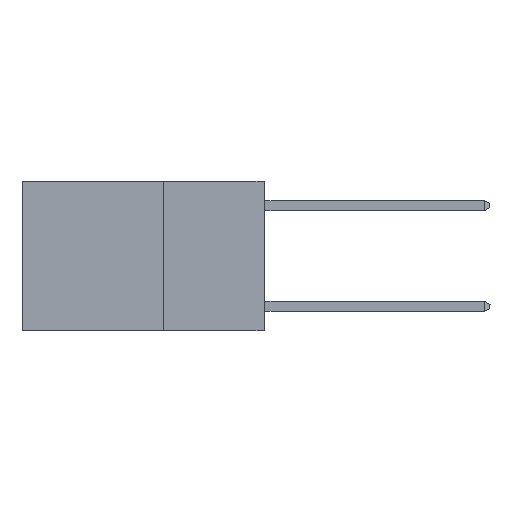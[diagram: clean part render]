
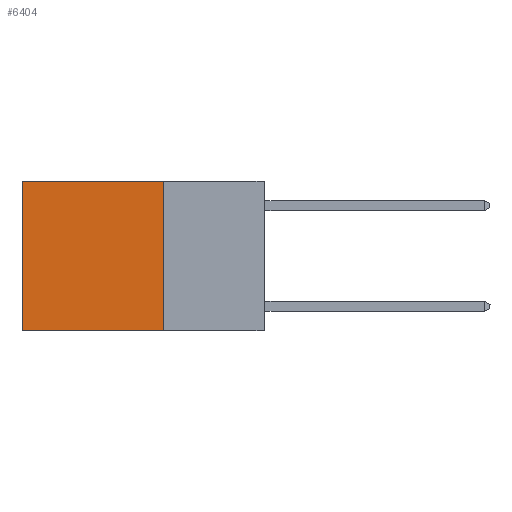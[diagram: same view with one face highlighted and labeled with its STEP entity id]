
A CAD part, left-side view. The second image highlights one B-rep face of the part: STEP entity #6404.
In plain terms, the highlighted planar face has unit normal (-1, 0, 0).
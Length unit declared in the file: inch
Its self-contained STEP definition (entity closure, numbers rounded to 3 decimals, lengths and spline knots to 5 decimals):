
#98 = EDGE_CURVE ( 'NONE', #1555, #681, #8851, .T. ) ;
#681 = VERTEX_POINT ( 'NONE', #6978 ) ;
#824 = EDGE_LOOP ( 'NONE', ( #1961, #2240, #9434, #9918 ) ) ;
#958 = VERTEX_POINT ( 'NONE', #6977 ) ;
#1031 = DIRECTION ( 'NONE',  ( 0., 0., -1. ) ) ;
#1322 = EDGE_CURVE ( 'NONE', #7547, #1555, #7709, .T. ) ;
#1414 = CARTESIAN_POINT ( 'NONE',  ( 0.2625, 0.6, 0. ) ) ;
#1555 = VERTEX_POINT ( 'NONE', #6899 ) ;
#1961 = ORIENTED_EDGE ( 'NONE', *, *, #9057, .T. ) ;
#2240 = ORIENTED_EDGE ( 'NONE', *, *, #98, .F. ) ;
#2526 = CARTESIAN_POINT ( 'NONE',  ( 0.2625, 0.25, -0.37 ) ) ;
#3001 = CARTESIAN_POINT ( 'NONE',  ( 0.2625, 0.25, 0. ) ) ;
#3816 = VECTOR ( 'NONE', #6089, 39.37008 ) ;
#4702 = CARTESIAN_POINT ( 'NONE',  ( 0.2625, 0.25, 0. ) ) ;
#4886 = VECTOR ( 'NONE', #12712, 39.37008 ) ;
#5017 = PLANE ( 'NONE',  #7343 ) ;
#5266 = VECTOR ( 'NONE', #12694, 39.37008 ) ;
#6089 = DIRECTION ( 'NONE',  ( 0., 1., 0. ) ) ;
#6404 = ADVANCED_FACE ( 'NONE', ( #6633 ), #5017, .F. ) ;
#6525 = LINE ( 'NONE', #12337, #3816 ) ;
#6633 = FACE_OUTER_BOUND ( 'NONE', #824, .T. ) ;
#6899 = CARTESIAN_POINT ( 'NONE',  ( 0.2625, 0.25, -0.37 ) ) ;
#6977 = CARTESIAN_POINT ( 'NONE',  ( 0.2625, 0.6, 0. ) ) ;
#6978 = CARTESIAN_POINT ( 'NONE',  ( 0.2625, 0.6, -0.37 ) ) ;
#7101 = DIRECTION ( 'NONE',  ( 1., 0., 0. ) ) ;
#7343 = AXIS2_PLACEMENT_3D ( 'NONE', #3001, #7101, #1031 ) ;
#7547 = VERTEX_POINT ( 'NONE', #4702 ) ;
#7688 = VECTOR ( 'NONE', #11388, 39.37008 ) ;
#7709 = LINE ( 'NONE', #11270, #7688 ) ;
#8263 = EDGE_CURVE ( 'NONE', #7547, #958, #6525, .T. ) ;
#8851 = LINE ( 'NONE', #2526, #4886 ) ;
#9057 = EDGE_CURVE ( 'NONE', #958, #681, #10827, .T. ) ;
#9434 = ORIENTED_EDGE ( 'NONE', *, *, #1322, .F. ) ;
#9918 = ORIENTED_EDGE ( 'NONE', *, *, #8263, .T. ) ;
#10827 = LINE ( 'NONE', #1414, #5266 ) ;
#11270 = CARTESIAN_POINT ( 'NONE',  ( 0.2625, 0.25, 0. ) ) ;
#11388 = DIRECTION ( 'NONE',  ( 0., 0., -1. ) ) ;
#12337 = CARTESIAN_POINT ( 'NONE',  ( 0.2625, 0.25, 0. ) ) ;
#12694 = DIRECTION ( 'NONE',  ( 0., 0., -1. ) ) ;
#12712 = DIRECTION ( 'NONE',  ( 0., 1., 0. ) ) ;
